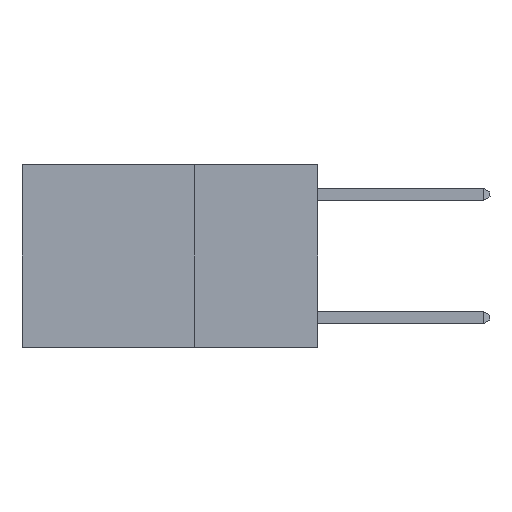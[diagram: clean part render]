
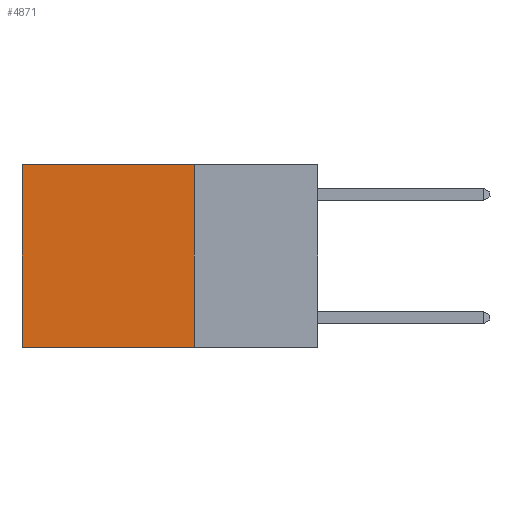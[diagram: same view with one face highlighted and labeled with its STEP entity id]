
A CAD part, left-side view. The second image highlights one B-rep face of the part: STEP entity #4871.
In plain terms, the highlighted planar face has unit normal (-1, 0, 0).
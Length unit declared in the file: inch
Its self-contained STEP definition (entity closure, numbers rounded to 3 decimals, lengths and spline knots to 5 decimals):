
#1 = CARTESIAN_POINT ( 'NONE',  ( 0.2625, 0.6, 0. ) ) ;
#29 = DIRECTION ( 'NONE',  ( 0., 1., 0. ) ) ;
#120 = VERTEX_POINT ( 'NONE', #6304 ) ;
#170 = PLANE ( 'NONE',  #7585 ) ;
#405 = DIRECTION ( 'NONE',  ( 0., 0., -1. ) ) ;
#760 = VERTEX_POINT ( 'NONE', #5099 ) ;
#891 = ORIENTED_EDGE ( 'NONE', *, *, #1520, .F. ) ;
#1018 = DIRECTION ( 'NONE',  ( 0., 0., -1. ) ) ;
#1520 = EDGE_CURVE ( 'NONE', #760, #120, #2969, .T. ) ;
#1818 = VERTEX_POINT ( 'NONE', #3593 ) ;
#1954 = DIRECTION ( 'NONE',  ( 0., 1., 0. ) ) ;
#2969 = LINE ( 'NONE', #7359, #7727 ) ;
#2999 = ORIENTED_EDGE ( 'NONE', *, *, #4026, .F. ) ;
#3593 = CARTESIAN_POINT ( 'NONE',  ( 0.2625, 0.25, 0. ) ) ;
#3601 = VERTEX_POINT ( 'NONE', #7783 ) ;
#3608 = EDGE_CURVE ( 'NONE', #1818, #3601, #5622, .T. ) ;
#4026 = EDGE_CURVE ( 'NONE', #1818, #760, #8593, .T. ) ;
#4454 = DIRECTION ( 'NONE',  ( 0., 0., -1. ) ) ;
#4871 = ADVANCED_FACE ( 'NONE', ( #8232 ), #170, .F. ) ;
#4964 = EDGE_LOOP ( 'NONE', ( #6168, #891, #2999, #8152 ) ) ;
#5099 = CARTESIAN_POINT ( 'NONE',  ( 0.2625, 0.25, -0.37 ) ) ;
#5190 = VECTOR ( 'NONE', #1018, 39.37008 ) ;
#5226 = LINE ( 'NONE', #1, #8881 ) ;
#5353 = CARTESIAN_POINT ( 'NONE',  ( 0.2625, 0.25, 0. ) ) ;
#5523 = CARTESIAN_POINT ( 'NONE',  ( 0.2625, 0.25, 0. ) ) ;
#5622 = LINE ( 'NONE', #8559, #8705 ) ;
#5791 = EDGE_CURVE ( 'NONE', #3601, #120, #5226, .T. ) ;
#6168 = ORIENTED_EDGE ( 'NONE', *, *, #5791, .T. ) ;
#6304 = CARTESIAN_POINT ( 'NONE',  ( 0.2625, 0.6, -0.37 ) ) ;
#7359 = CARTESIAN_POINT ( 'NONE',  ( 0.2625, 0.25, -0.37 ) ) ;
#7585 = AXIS2_PLACEMENT_3D ( 'NONE', #5353, #8282, #405 ) ;
#7727 = VECTOR ( 'NONE', #29, 39.37008 ) ;
#7783 = CARTESIAN_POINT ( 'NONE',  ( 0.2625, 0.6, 0. ) ) ;
#8152 = ORIENTED_EDGE ( 'NONE', *, *, #3608, .T. ) ;
#8232 = FACE_OUTER_BOUND ( 'NONE', #4964, .T. ) ;
#8282 = DIRECTION ( 'NONE',  ( 1., 0., 0. ) ) ;
#8559 = CARTESIAN_POINT ( 'NONE',  ( 0.2625, 0.25, 0. ) ) ;
#8593 = LINE ( 'NONE', #5523, #5190 ) ;
#8705 = VECTOR ( 'NONE', #1954, 39.37008 ) ;
#8881 = VECTOR ( 'NONE', #4454, 39.37008 ) ;
